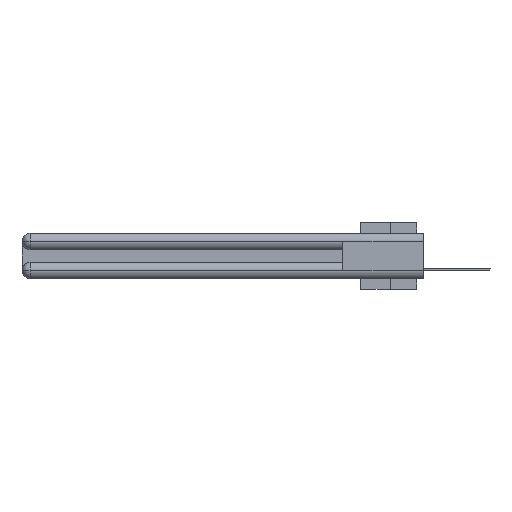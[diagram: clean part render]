
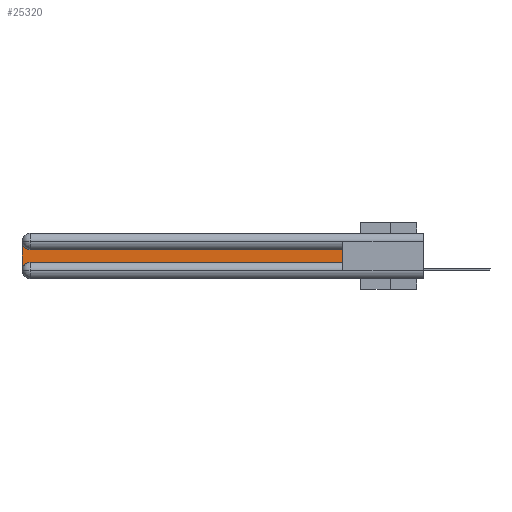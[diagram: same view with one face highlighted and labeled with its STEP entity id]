
A CAD part, left-side view. The second image highlights one B-rep face of the part: STEP entity #25320.
In plain terms, the highlighted planar face has unit normal (-1, 0, 0).
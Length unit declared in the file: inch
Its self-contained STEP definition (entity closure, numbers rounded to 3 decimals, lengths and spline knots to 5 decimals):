
#157 = CIRCLE ( 'NONE', #32931, 0.06 ) ;
#278 = CARTESIAN_POINT ( 'NONE',  ( 0.075, 0.6, -0.2175 ) ) ;
#298 = VECTOR ( 'NONE', #22682, 39.37008 ) ;
#520 = CARTESIAN_POINT ( 'NONE',  ( 0.075, 3., -0.2175 ) ) ;
#992 = VERTEX_POINT ( 'NONE', #278 ) ;
#1594 = EDGE_CURVE ( 'NONE', #9674, #14923, #27973, .T. ) ;
#3729 = CARTESIAN_POINT ( 'NONE',  ( 0.075, 0.6, -0.1225 ) ) ;
#5288 = DIRECTION ( 'NONE',  ( 1., 0., 0. ) ) ;
#8326 = ORIENTED_EDGE ( 'NONE', *, *, #11135, .T. ) ;
#8517 = VERTEX_POINT ( 'NONE', #24530 ) ;
#8827 = DIRECTION ( 'NONE',  ( 0., 0., -1. ) ) ;
#9674 = VERTEX_POINT ( 'NONE', #15178 ) ;
#9907 = ORIENTED_EDGE ( 'NONE', *, *, #1594, .T. ) ;
#10422 = CARTESIAN_POINT ( 'NONE',  ( 0.075, 2.94, -0.2775 ) ) ;
#10585 = DIRECTION ( 'NONE',  ( 0., -1., 0. ) ) ;
#10984 = CIRCLE ( 'NONE', #22886, 0.06 ) ;
#11135 = EDGE_CURVE ( 'NONE', #8517, #992, #13240, .T. ) ;
#13217 = DIRECTION ( 'NONE',  ( 1., 0., 0. ) ) ;
#13240 = LINE ( 'NONE', #24071, #20271 ) ;
#13881 = CARTESIAN_POINT ( 'NONE',  ( 0.075, 3., -0.0625 ) ) ;
#14087 = AXIS2_PLACEMENT_3D ( 'NONE', #24529, #32463, #34768 ) ;
#14568 = CARTESIAN_POINT ( 'NONE',  ( 0.075, 3., -0.2775 ) ) ;
#14574 = CARTESIAN_POINT ( 'NONE',  ( 0.075, 0.6, -0.2175 ) ) ;
#14923 = VERTEX_POINT ( 'NONE', #17824 ) ;
#15178 = CARTESIAN_POINT ( 'NONE',  ( 0.075, 0.6, -0.1225 ) ) ;
#17824 = CARTESIAN_POINT ( 'NONE',  ( 0.075, 2.94, -0.1225 ) ) ;
#18714 = DIRECTION ( 'NONE',  ( 0., 0., -1. ) ) ;
#19118 = EDGE_CURVE ( 'NONE', #14923, #29673, #10984, .T. ) ;
#19551 = DIRECTION ( 'NONE',  ( 0., 0., 1. ) ) ;
#19640 = LINE ( 'NONE', #520, #28129 ) ;
#19839 = VERTEX_POINT ( 'NONE', #14568 ) ;
#20271 = VECTOR ( 'NONE', #10585, 39.37008 ) ;
#20713 = ORIENTED_EDGE ( 'NONE', *, *, #25369, .T. ) ;
#21226 = DIRECTION ( 'NONE',  ( 0., 0., -1. ) ) ;
#21684 = FACE_OUTER_BOUND ( 'NONE', #29914, .T. ) ;
#22121 = EDGE_CURVE ( 'NONE', #29673, #19839, #19640, .T. ) ;
#22682 = DIRECTION ( 'NONE',  ( 0., 1., 0. ) ) ;
#22886 = AXIS2_PLACEMENT_3D ( 'NONE', #28976, #13217, #18714 ) ;
#23869 = ORIENTED_EDGE ( 'NONE', *, *, #32099, .T. ) ;
#23978 = ORIENTED_EDGE ( 'NONE', *, *, #19118, .T. ) ;
#24015 = PLANE ( 'NONE',  #14087 ) ;
#24071 = CARTESIAN_POINT ( 'NONE',  ( 0.075, 0.6, -0.2175 ) ) ;
#24529 = CARTESIAN_POINT ( 'NONE',  ( 0.075, 3., -0.1225 ) ) ;
#24530 = CARTESIAN_POINT ( 'NONE',  ( 0.075, 2.94, -0.2175 ) ) ;
#24998 = ORIENTED_EDGE ( 'NONE', *, *, #22121, .T. ) ;
#25320 = ADVANCED_FACE ( 'NONE', ( #21684 ), #24015, .F. ) ;
#25369 = EDGE_CURVE ( 'NONE', #992, #9674, #30335, .T. ) ;
#27973 = LINE ( 'NONE', #3729, #298 ) ;
#28129 = VECTOR ( 'NONE', #8827, 39.37008 ) ;
#28796 = VECTOR ( 'NONE', #19551, 39.37008 ) ;
#28976 = CARTESIAN_POINT ( 'NONE',  ( 0.075, 2.94, -0.0625 ) ) ;
#29673 = VERTEX_POINT ( 'NONE', #13881 ) ;
#29914 = EDGE_LOOP ( 'NONE', ( #9907, #23978, #24998, #23869, #8326, #20713 ) ) ;
#30335 = LINE ( 'NONE', #14574, #28796 ) ;
#32099 = EDGE_CURVE ( 'NONE', #19839, #8517, #157, .T. ) ;
#32463 = DIRECTION ( 'NONE',  ( 1., 0., 0. ) ) ;
#32931 = AXIS2_PLACEMENT_3D ( 'NONE', #10422, #5288, #21226 ) ;
#34768 = DIRECTION ( 'NONE',  ( 0., 0., -1. ) ) ;
